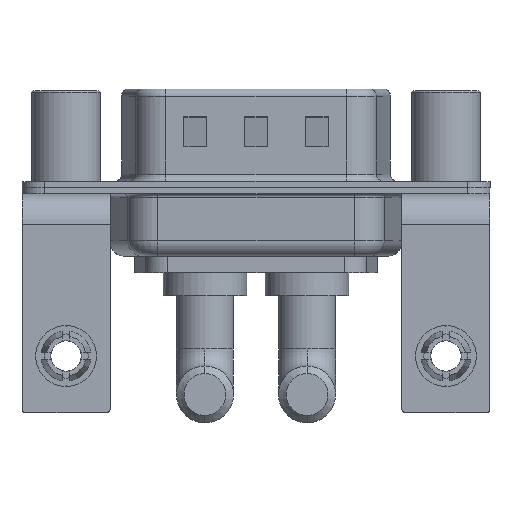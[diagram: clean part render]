
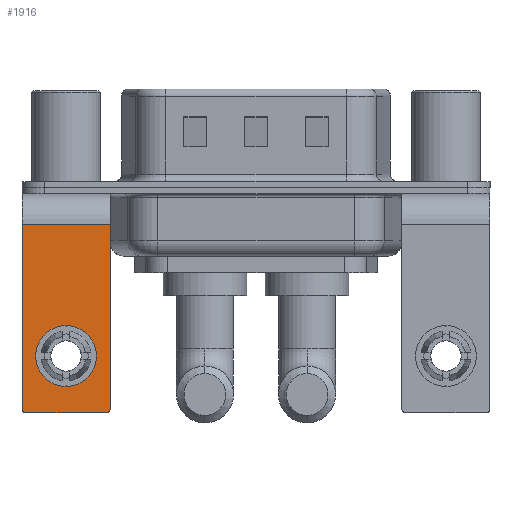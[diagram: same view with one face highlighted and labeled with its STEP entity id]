
A CAD part, front view. The second image highlights one B-rep face of the part: STEP entity #1916.
In plain terms, the highlighted planar face has unit normal (0, -1, 0).
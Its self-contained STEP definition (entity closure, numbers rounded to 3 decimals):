
#244 = CARTESIAN_POINT ( 'NONE',  ( -2.9, -6.25, -2.4 ) ) ;
#297 = DIRECTION ( 'NONE',  ( 0., 0., 1. ) ) ;
#321 = DIRECTION ( 'NONE',  ( 0., -1., 0. ) ) ;
#340 = DIRECTION ( 'NONE',  ( 0., 0., -1. ) ) ;
#531 = CARTESIAN_POINT ( 'NONE',  ( 2.9, -6.25, -14.8 ) ) ;
#1537 = EDGE_CURVE ( 'NONE', #16338, #16551, #8827, .T. ) ;
#1756 = VERTEX_POINT ( 'NONE', #8266 ) ;
#1916 = ADVANCED_FACE ( 'NONE', ( #14146, #7010 ), #15334, .F. ) ;
#2070 = LINE ( 'NONE', #2575, #15362 ) ;
#2394 = EDGE_CURVE ( 'NONE', #2662, #1756, #9801, .T. ) ;
#2575 = CARTESIAN_POINT ( 'NONE',  ( 2.9, -6.25, -2.4 ) ) ;
#2596 = DIRECTION ( 'NONE',  ( 0., 0., 1. ) ) ;
#2662 = VERTEX_POINT ( 'NONE', #6243 ) ;
#2714 = CARTESIAN_POINT ( 'NONE',  ( -2.9, -6.25, -2.4 ) ) ;
#3071 = EDGE_CURVE ( 'NONE', #11217, #12819, #8485, .T. ) ;
#3218 = DIRECTION ( 'NONE',  ( 0., 1., 0. ) ) ;
#3294 = EDGE_CURVE ( 'NONE', #1756, #2662, #8398, .T. ) ;
#3311 = DIRECTION ( 'NONE',  ( 0., 0., 1. ) ) ;
#3386 = ORIENTED_EDGE ( 'NONE', *, *, #3294, .T. ) ;
#3437 = CIRCLE ( 'NONE', #13249, 0.25 ) ;
#4082 = DIRECTION ( 'NONE',  ( 0., 0., -1. ) ) ;
#4319 = CARTESIAN_POINT ( 'NONE',  ( 2.65, -6.25, -14.8 ) ) ;
#4691 = CARTESIAN_POINT ( 'NONE',  ( 2.9, -6.25, -2.4 ) ) ;
#4706 = DIRECTION ( 'NONE',  ( -1., 0., 0. ) ) ;
#5225 = ORIENTED_EDGE ( 'NONE', *, *, #17655, .T. ) ;
#5644 = DIRECTION ( 'NONE',  ( 0., 1., 0. ) ) ;
#6045 = DIRECTION ( 'NONE',  ( -1., 0., 0. ) ) ;
#6203 = CARTESIAN_POINT ( 'NONE',  ( -2.9, -6.25, -14.55 ) ) ;
#6243 = CARTESIAN_POINT ( 'NONE',  ( 0., -6.25, -13.07 ) ) ;
#6314 = AXIS2_PLACEMENT_3D ( 'NONE', #15515, #3218, #3311 ) ;
#6351 = AXIS2_PLACEMENT_3D ( 'NONE', #7163, #5644, #297 ) ;
#6845 = CARTESIAN_POINT ( 'NONE',  ( 2.9, -6.25, -14.55 ) ) ;
#6930 = DIRECTION ( 'NONE',  ( 0., -1., 0. ) ) ;
#7010 = FACE_OUTER_BOUND ( 'NONE', #15965, .T. ) ;
#7163 = CARTESIAN_POINT ( 'NONE',  ( 0., -6.25, -11.07 ) ) ;
#7408 = ORIENTED_EDGE ( 'NONE', *, *, #15137, .T. ) ;
#8266 = CARTESIAN_POINT ( 'NONE',  ( 0., -6.25, -9.07 ) ) ;
#8398 = CIRCLE ( 'NONE', #15331, 2. ) ;
#8448 = DIRECTION ( 'NONE',  ( 0., 0., 1. ) ) ;
#8485 = LINE ( 'NONE', #2714, #11570 ) ;
#8622 = CARTESIAN_POINT ( 'NONE',  ( 2.65, -6.25, -14.55 ) ) ;
#8827 = LINE ( 'NONE', #4691, #11116 ) ;
#9035 = ORIENTED_EDGE ( 'NONE', *, *, #9433, .F. ) ;
#9101 = VECTOR ( 'NONE', #6045, 1000. ) ;
#9420 = ORIENTED_EDGE ( 'NONE', *, *, #1537, .F. ) ;
#9433 = EDGE_CURVE ( 'NONE', #9772, #14327, #12908, .T. ) ;
#9494 = AXIS2_PLACEMENT_3D ( 'NONE', #12333, #6930, #2596 ) ;
#9772 = VERTEX_POINT ( 'NONE', #4319 ) ;
#9801 = CIRCLE ( 'NONE', #6351, 2. ) ;
#10472 = ORIENTED_EDGE ( 'NONE', *, *, #2394, .T. ) ;
#11116 = VECTOR ( 'NONE', #340, 1000. ) ;
#11217 = VERTEX_POINT ( 'NONE', #244 ) ;
#11570 = VECTOR ( 'NONE', #4082, 1000. ) ;
#12034 = EDGE_LOOP ( 'NONE', ( #10472, #3386 ) ) ;
#12333 = CARTESIAN_POINT ( 'NONE',  ( -2.65, -6.25, -14.55 ) ) ;
#12729 = CARTESIAN_POINT ( 'NONE',  ( 0., -6.25, -11.07 ) ) ;
#12819 = VERTEX_POINT ( 'NONE', #6203 ) ;
#12908 = LINE ( 'NONE', #531, #9101 ) ;
#13096 = EDGE_CURVE ( 'NONE', #9772, #16551, #3437, .T. ) ;
#13249 = AXIS2_PLACEMENT_3D ( 'NONE', #8622, #321, #8448 ) ;
#13537 = CIRCLE ( 'NONE', #9494, 0.25 ) ;
#14037 = CARTESIAN_POINT ( 'NONE',  ( -2.65, -6.25, -14.8 ) ) ;
#14146 = FACE_BOUND ( 'NONE', #12034, .T. ) ;
#14269 = DIRECTION ( 'NONE',  ( 0., 0., 1. ) ) ;
#14327 = VERTEX_POINT ( 'NONE', #14037 ) ;
#15137 = EDGE_CURVE ( 'NONE', #12819, #14327, #13537, .T. ) ;
#15311 = ORIENTED_EDGE ( 'NONE', *, *, #13096, .T. ) ;
#15331 = AXIS2_PLACEMENT_3D ( 'NONE', #12729, #15640, #14269 ) ;
#15334 = PLANE ( 'NONE',  #6314 ) ;
#15362 = VECTOR ( 'NONE', #4706, 1000. ) ;
#15515 = CARTESIAN_POINT ( 'NONE',  ( 2.9, -6.25, -2.4 ) ) ;
#15640 = DIRECTION ( 'NONE',  ( 0., 1., 0. ) ) ;
#15965 = EDGE_LOOP ( 'NONE', ( #16012, #7408, #9035, #15311, #9420, #5225 ) ) ;
#16012 = ORIENTED_EDGE ( 'NONE', *, *, #3071, .T. ) ;
#16338 = VERTEX_POINT ( 'NONE', #16715 ) ;
#16551 = VERTEX_POINT ( 'NONE', #6845 ) ;
#16715 = CARTESIAN_POINT ( 'NONE',  ( 2.9, -6.25, -2.4 ) ) ;
#17655 = EDGE_CURVE ( 'NONE', #16338, #11217, #2070, .T. ) ;
